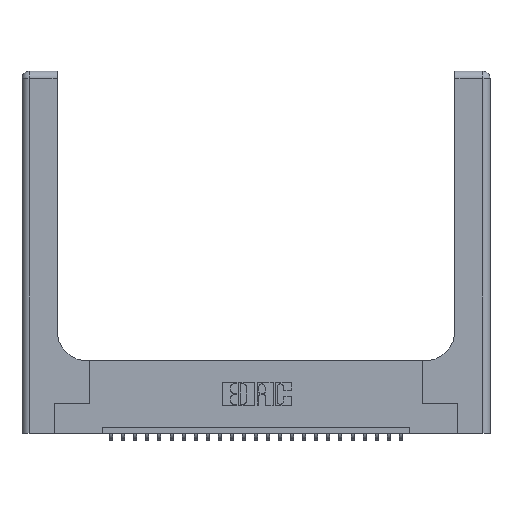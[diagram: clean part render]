
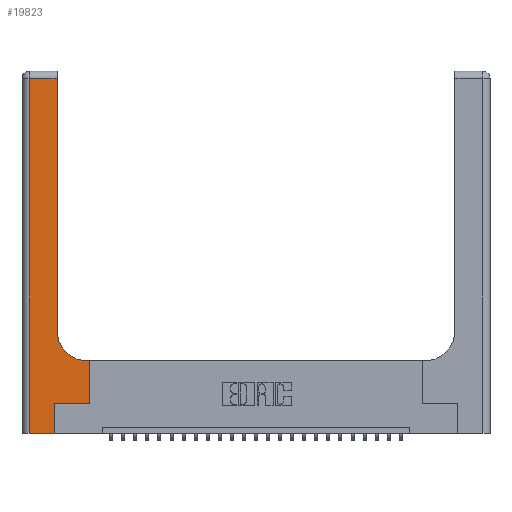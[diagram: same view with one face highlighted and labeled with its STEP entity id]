
A CAD part, top view. The second image highlights one B-rep face of the part: STEP entity #19823.
In plain terms, the highlighted planar face has unit normal (0, 0, 1).
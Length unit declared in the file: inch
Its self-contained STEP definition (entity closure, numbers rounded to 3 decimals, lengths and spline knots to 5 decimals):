
#584 = ORIENTED_EDGE ( 'NONE', *, *, #23984, .T. ) ;
#605 = LINE ( 'NONE', #16911, #14921 ) ;
#1360 = DIRECTION ( 'NONE',  ( 0., -1., 0. ) ) ;
#1433 = CARTESIAN_POINT ( 'NONE',  ( 0., 3., 0.37 ) ) ;
#1596 = CARTESIAN_POINT ( 'NONE',  ( 0., 0., 0.37 ) ) ;
#1605 = CARTESIAN_POINT ( 'NONE',  ( 0.06, 0., 0.37 ) ) ;
#4710 = DIRECTION ( 'NONE',  ( 0., 1., 0. ) ) ;
#5204 = VECTOR ( 'NONE', #16243, 39.37008 ) ;
#5258 = DIRECTION ( 'NONE',  ( -1., 0., 0. ) ) ;
#5321 = CARTESIAN_POINT ( 'NONE',  ( 0.5585, 0.6, 0.37 ) ) ;
#5355 = DIRECTION ( 'NONE',  ( 1., 0., 0. ) ) ;
#5663 = VERTEX_POINT ( 'NONE', #9849 ) ;
#5692 = VECTOR ( 'NONE', #8305, 39.37008 ) ;
#5999 = AXIS2_PLACEMENT_3D ( 'NONE', #1433, #9625, #5258 ) ;
#6659 = CARTESIAN_POINT ( 'NONE',  ( 0., 2.94, 0.37 ) ) ;
#6704 = DIRECTION ( 'NONE',  ( 0., 1., 0. ) ) ;
#6964 = VERTEX_POINT ( 'NONE', #14785 ) ;
#7296 = CARTESIAN_POINT ( 'NONE',  ( 0.269, 0., 0.37 ) ) ;
#7322 = EDGE_CURVE ( 'NONE', #19932, #16059, #20043, .T. ) ;
#7335 = ORIENTED_EDGE ( 'NONE', *, *, #7322, .T. ) ;
#7523 = VECTOR ( 'NONE', #24175, 39.37008 ) ;
#7551 = LINE ( 'NONE', #10759, #25031 ) ;
#7921 = CARTESIAN_POINT ( 'NONE',  ( 0.5585, 0.25, 0.37 ) ) ;
#8305 = DIRECTION ( 'NONE',  ( 1., 0., 0. ) ) ;
#8780 = LINE ( 'NONE', #7921, #7523 ) ;
#9203 = VERTEX_POINT ( 'NONE', #26162 ) ;
#9374 = DIRECTION ( 'NONE',  ( 0., 0., -1. ) ) ;
#9465 = PLANE ( 'NONE',  #5999 ) ;
#9625 = DIRECTION ( 'NONE',  ( 0., 0., -1. ) ) ;
#9849 = CARTESIAN_POINT ( 'NONE',  ( 0.06, 2.94, 0.37 ) ) ;
#9924 = CARTESIAN_POINT ( 'NONE',  ( 0.2915, 2.94, 0.37 ) ) ;
#10197 = EDGE_CURVE ( 'NONE', #16059, #24076, #605, .T. ) ;
#10220 = VECTOR ( 'NONE', #6704, 39.37008 ) ;
#10759 = CARTESIAN_POINT ( 'NONE',  ( 0.269, 0.25, 0.37 ) ) ;
#13004 = EDGE_CURVE ( 'NONE', #19269, #5663, #21487, .T. ) ;
#13055 = VERTEX_POINT ( 'NONE', #5321 ) ;
#13198 = EDGE_CURVE ( 'NONE', #13055, #25194, #17310, .T. ) ;
#13429 = ORIENTED_EDGE ( 'NONE', *, *, #23526, .T. ) ;
#13469 = ORIENTED_EDGE ( 'NONE', *, *, #10197, .T. ) ;
#14777 = CARTESIAN_POINT ( 'NONE',  ( 0.2915, 3., 0.37 ) ) ;
#14785 = CARTESIAN_POINT ( 'NONE',  ( 0.2915, 0.85, 0.37 ) ) ;
#14792 = CARTESIAN_POINT ( 'NONE',  ( 0.5415, 0.6, 0.37 ) ) ;
#14921 = VECTOR ( 'NONE', #4710, 39.37008 ) ;
#15536 = AXIS2_PLACEMENT_3D ( 'NONE', #23779, #9374, #5355 ) ;
#16059 = VERTEX_POINT ( 'NONE', #7296 ) ;
#16243 = DIRECTION ( 'NONE',  ( -1., 0., 0. ) ) ;
#16687 = VECTOR ( 'NONE', #25577, 39.37008 ) ;
#16911 = CARTESIAN_POINT ( 'NONE',  ( 0.269, 0., 0.37 ) ) ;
#17310 = LINE ( 'NONE', #20291, #5204 ) ;
#17836 = ORIENTED_EDGE ( 'NONE', *, *, #13004, .T. ) ;
#18774 = CARTESIAN_POINT ( 'NONE',  ( 0.269, 0.25, 0.37 ) ) ;
#19001 = ORIENTED_EDGE ( 'NONE', *, *, #25467, .T. ) ;
#19269 = VERTEX_POINT ( 'NONE', #9924 ) ;
#19592 = EDGE_CURVE ( 'NONE', #6964, #19269, #23262, .T. ) ;
#19748 = EDGE_CURVE ( 'NONE', #25194, #6964, #22312, .T. ) ;
#19823 = ADVANCED_FACE ( 'NONE', ( #24824 ), #9465, .F. ) ;
#19932 = VERTEX_POINT ( 'NONE', #1605 ) ;
#19964 = CARTESIAN_POINT ( 'NONE',  ( 0.06, 3., 0.37 ) ) ;
#20043 = LINE ( 'NONE', #1596, #5692 ) ;
#20291 = CARTESIAN_POINT ( 'NONE',  ( 0.2915, 0.6, 0.37 ) ) ;
#20340 = EDGE_LOOP ( 'NONE', ( #23692, #17836, #19001, #7335, #13469, #13429, #584, #23398, #26234 ) ) ;
#21487 = LINE ( 'NONE', #6659, #16687 ) ;
#22312 = CIRCLE ( 'NONE', #15536, 0.25 ) ;
#22861 = DIRECTION ( 'NONE',  ( 1., 0., 0. ) ) ;
#22998 = VECTOR ( 'NONE', #1360, 39.37008 ) ;
#23262 = LINE ( 'NONE', #14777, #10220 ) ;
#23398 = ORIENTED_EDGE ( 'NONE', *, *, #13198, .T. ) ;
#23526 = EDGE_CURVE ( 'NONE', #24076, #9203, #7551, .T. ) ;
#23692 = ORIENTED_EDGE ( 'NONE', *, *, #19592, .T. ) ;
#23779 = CARTESIAN_POINT ( 'NONE',  ( 0.5415, 0.85, 0.37 ) ) ;
#23984 = EDGE_CURVE ( 'NONE', #9203, #13055, #8780, .T. ) ;
#24076 = VERTEX_POINT ( 'NONE', #18774 ) ;
#24175 = DIRECTION ( 'NONE',  ( 0., 1., 0. ) ) ;
#24591 = LINE ( 'NONE', #19964, #22998 ) ;
#24824 = FACE_OUTER_BOUND ( 'NONE', #20340, .T. ) ;
#25031 = VECTOR ( 'NONE', #22861, 39.37008 ) ;
#25194 = VERTEX_POINT ( 'NONE', #14792 ) ;
#25467 = EDGE_CURVE ( 'NONE', #5663, #19932, #24591, .T. ) ;
#25577 = DIRECTION ( 'NONE',  ( -1., 0., 0. ) ) ;
#26162 = CARTESIAN_POINT ( 'NONE',  ( 0.5585, 0.25, 0.37 ) ) ;
#26234 = ORIENTED_EDGE ( 'NONE', *, *, #19748, .T. ) ;
